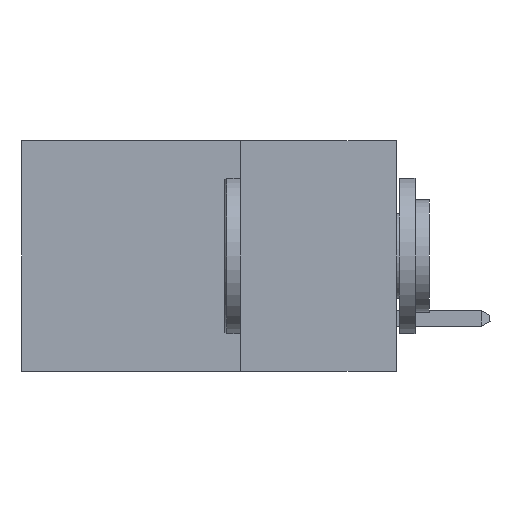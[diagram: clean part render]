
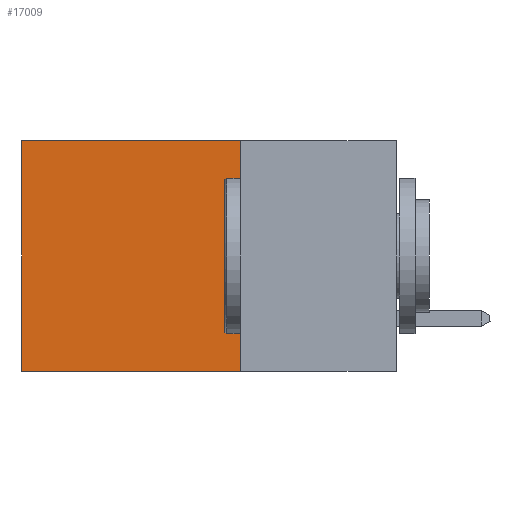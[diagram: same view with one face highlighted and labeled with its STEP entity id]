
A CAD part, left-side view. The second image highlights one B-rep face of the part: STEP entity #17009.
In plain terms, the highlighted planar face has unit normal (-1, 0, 0).
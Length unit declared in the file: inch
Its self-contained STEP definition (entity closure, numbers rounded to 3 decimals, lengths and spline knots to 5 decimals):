
#827 = LINE ( 'NONE', #6853, #15143 ) ;
#1011 = CARTESIAN_POINT ( 'NONE',  ( 0.298, 0.25, 0. ) ) ;
#1069 = EDGE_CURVE ( 'NONE', #4126, #1491, #1899, .T. ) ;
#1491 = VERTEX_POINT ( 'NONE', #12808 ) ;
#1736 = PLANE ( 'NONE',  #13516 ) ;
#1899 = LINE ( 'NONE', #1011, #5459 ) ;
#2216 = VECTOR ( 'NONE', #10101, 39.37008 ) ;
#2683 = LINE ( 'NONE', #15525, #2216 ) ;
#3571 = CARTESIAN_POINT ( 'NONE',  ( 0.298, 0.6, -0.37 ) ) ;
#4126 = VERTEX_POINT ( 'NONE', #12639 ) ;
#4228 = EDGE_CURVE ( 'NONE', #1491, #6841, #2683, .T. ) ;
#4260 = ORIENTED_EDGE ( 'NONE', *, *, #1069, .T. ) ;
#4781 = DIRECTION ( 'NONE',  ( 1., 0., 0. ) ) ;
#5063 = CARTESIAN_POINT ( 'NONE',  ( 0.298, 0.25, 0. ) ) ;
#5459 = VECTOR ( 'NONE', #17342, 39.37008 ) ;
#6304 = LINE ( 'NONE', #5063, #17389 ) ;
#6841 = VERTEX_POINT ( 'NONE', #3571 ) ;
#6853 = CARTESIAN_POINT ( 'NONE',  ( 0.298, 0.25, -0.37 ) ) ;
#7181 = ORIENTED_EDGE ( 'NONE', *, *, #11027, .F. ) ;
#7764 = EDGE_LOOP ( 'NONE', ( #10921, #7181, #10494, #4260 ) ) ;
#8285 = DIRECTION ( 'NONE',  ( 0., 1., 0. ) ) ;
#10101 = DIRECTION ( 'NONE',  ( 0., 0., -1. ) ) ;
#10494 = ORIENTED_EDGE ( 'NONE', *, *, #14653, .F. ) ;
#10516 = CARTESIAN_POINT ( 'NONE',  ( 0.298, 0.25, 0. ) ) ;
#10921 = ORIENTED_EDGE ( 'NONE', *, *, #4228, .T. ) ;
#11027 = EDGE_CURVE ( 'NONE', #17320, #6841, #827, .T. ) ;
#12639 = CARTESIAN_POINT ( 'NONE',  ( 0.298, 0.25, 0. ) ) ;
#12808 = CARTESIAN_POINT ( 'NONE',  ( 0.298, 0.6, 0. ) ) ;
#13516 = AXIS2_PLACEMENT_3D ( 'NONE', #10516, #4781, #14622 ) ;
#13607 = CARTESIAN_POINT ( 'NONE',  ( 0.298, 0.25, -0.37 ) ) ;
#13915 = FACE_OUTER_BOUND ( 'NONE', #7764, .T. ) ;
#14622 = DIRECTION ( 'NONE',  ( 0., 0., -1. ) ) ;
#14653 = EDGE_CURVE ( 'NONE', #4126, #17320, #6304, .T. ) ;
#14880 = DIRECTION ( 'NONE',  ( 0., 0., -1. ) ) ;
#15143 = VECTOR ( 'NONE', #8285, 39.37008 ) ;
#15525 = CARTESIAN_POINT ( 'NONE',  ( 0.298, 0.6, 0. ) ) ;
#17009 = ADVANCED_FACE ( 'NONE', ( #13915 ), #1736, .F. ) ;
#17320 = VERTEX_POINT ( 'NONE', #13607 ) ;
#17342 = DIRECTION ( 'NONE',  ( 0., 1., 0. ) ) ;
#17389 = VECTOR ( 'NONE', #14880, 39.37008 ) ;
